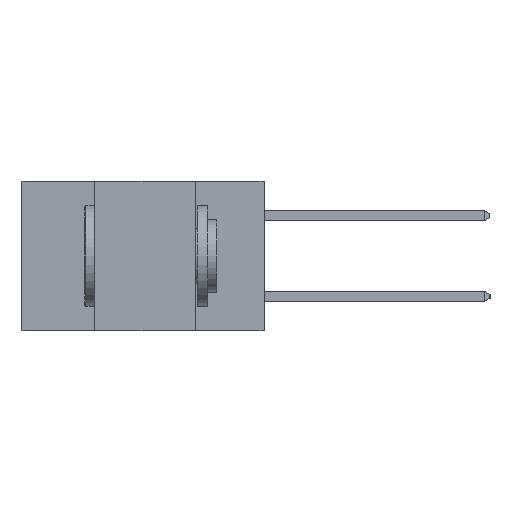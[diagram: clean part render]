
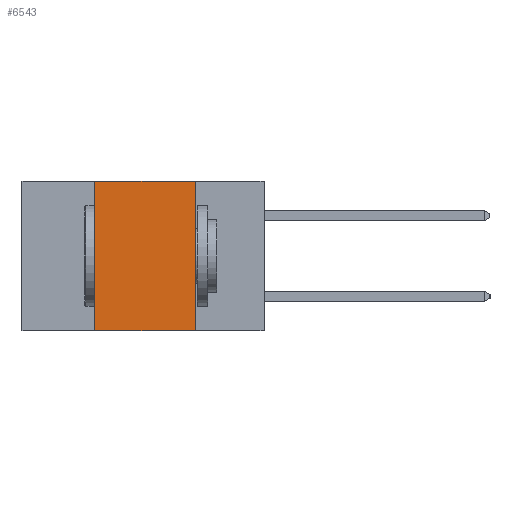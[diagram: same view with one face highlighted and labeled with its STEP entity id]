
A CAD part, left-side view. The second image highlights one B-rep face of the part: STEP entity #6543.
In plain terms, the highlighted planar face has unit normal (-1, 0, 0).
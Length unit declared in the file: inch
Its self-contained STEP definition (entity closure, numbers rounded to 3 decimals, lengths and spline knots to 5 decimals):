
#1427 = CARTESIAN_POINT ( 'NONE',  ( 0., 0.17, -0.37 ) ) ;
#1816 = ORIENTED_EDGE ( 'NONE', *, *, #8957, .F. ) ;
#2081 = VECTOR ( 'NONE', #15905, 39.37008 ) ;
#2325 = CARTESIAN_POINT ( 'NONE',  ( 0., 0.17, 0. ) ) ;
#2607 = LINE ( 'NONE', #20537, #2081 ) ;
#2619 = CARTESIAN_POINT ( 'NONE',  ( 0., 0.42, 0. ) ) ;
#2717 = CARTESIAN_POINT ( 'NONE',  ( 0., 0.6, -0.37 ) ) ;
#2861 = VERTEX_POINT ( 'NONE', #1427 ) ;
#4194 = LINE ( 'NONE', #11310, #12235 ) ;
#4344 = DIRECTION ( 'NONE',  ( 0., -1., 0. ) ) ;
#6283 = VERTEX_POINT ( 'NONE', #2325 ) ;
#6543 = ADVANCED_FACE ( 'NONE', ( #7942 ), #10834, .F. ) ;
#6709 = ORIENTED_EDGE ( 'NONE', *, *, #15115, .F. ) ;
#6936 = EDGE_CURVE ( 'NONE', #12332, #19544, #4194, .T. ) ;
#7942 = FACE_OUTER_BOUND ( 'NONE', #8099, .T. ) ;
#8099 = EDGE_LOOP ( 'NONE', ( #1816, #6709, #17021, #12102 ) ) ;
#8818 = DIRECTION ( 'NONE',  ( 0., -1., 0. ) ) ;
#8957 = EDGE_CURVE ( 'NONE', #6283, #2861, #2607, .T. ) ;
#8997 = VECTOR ( 'NONE', #4344, 39.37008 ) ;
#9815 = LINE ( 'NONE', #13658, #17722 ) ;
#10209 = CARTESIAN_POINT ( 'NONE',  ( 0., 0.6, 0. ) ) ;
#10834 = PLANE ( 'NONE',  #20223 ) ;
#11021 = DIRECTION ( 'NONE',  ( 0., 0., 1. ) ) ;
#11310 = CARTESIAN_POINT ( 'NONE',  ( 0., 0.42, -0.37 ) ) ;
#11590 = DIRECTION ( 'NONE',  ( 0., 0., -1. ) ) ;
#11678 = DIRECTION ( 'NONE',  ( 1., 0., 0. ) ) ;
#12102 = ORIENTED_EDGE ( 'NONE', *, *, #16929, .T. ) ;
#12235 = VECTOR ( 'NONE', #11021, 39.37008 ) ;
#12332 = VERTEX_POINT ( 'NONE', #12533 ) ;
#12533 = CARTESIAN_POINT ( 'NONE',  ( 0., 0.42, -0.37 ) ) ;
#13658 = CARTESIAN_POINT ( 'NONE',  ( 0., 0.6, 0. ) ) ;
#13784 = LINE ( 'NONE', #2717, #8997 ) ;
#15115 = EDGE_CURVE ( 'NONE', #19544, #6283, #9815, .T. ) ;
#15905 = DIRECTION ( 'NONE',  ( 0., 0., -1. ) ) ;
#16929 = EDGE_CURVE ( 'NONE', #12332, #2861, #13784, .T. ) ;
#17021 = ORIENTED_EDGE ( 'NONE', *, *, #6936, .F. ) ;
#17722 = VECTOR ( 'NONE', #8818, 39.37008 ) ;
#19544 = VERTEX_POINT ( 'NONE', #2619 ) ;
#20223 = AXIS2_PLACEMENT_3D ( 'NONE', #10209, #11678, #11590 ) ;
#20537 = CARTESIAN_POINT ( 'NONE',  ( 0., 0.17, -0.37 ) ) ;
